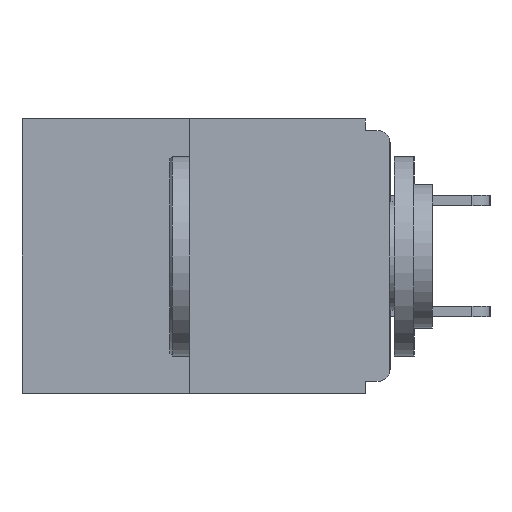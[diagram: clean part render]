
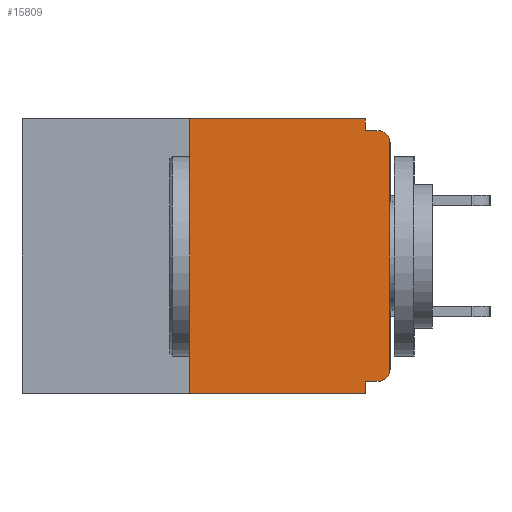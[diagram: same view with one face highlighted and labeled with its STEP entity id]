
A CAD part, left-side view. The second image highlights one B-rep face of the part: STEP entity #15809.
In plain terms, the highlighted planar face has unit normal (-1, 0, 0).
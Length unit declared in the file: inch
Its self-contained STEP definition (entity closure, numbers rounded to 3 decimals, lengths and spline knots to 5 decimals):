
#145 = VERTEX_POINT ( 'NONE', #18050 ) ;
#243 = VECTOR ( 'NONE', #1153, 39.37008 ) ;
#760 = CARTESIAN_POINT ( 'NONE',  ( 0., 0.015, -0.313 ) ) ;
#883 = AXIS2_PLACEMENT_3D ( 'NONE', #3754, #13693, #15143 ) ;
#996 = CARTESIAN_POINT ( 'NONE',  ( 0., 0.25, -0.343 ) ) ;
#1153 = DIRECTION ( 'NONE',  ( 0., -1., 0. ) ) ;
#1830 = AXIS2_PLACEMENT_3D ( 'NONE', #760, #5051, #13548 ) ;
#1889 = VECTOR ( 'NONE', #18510, 39.37008 ) ;
#1941 = CARTESIAN_POINT ( 'NONE',  ( 0., 0.46, 0. ) ) ;
#2300 = CARTESIAN_POINT ( 'NONE',  ( 0., 0., -0.328 ) ) ;
#2359 = EDGE_CURVE ( 'NONE', #15638, #13680, #3299, .T. ) ;
#2834 = CARTESIAN_POINT ( 'NONE',  ( 0., 0., 0. ) ) ;
#2894 = LINE ( 'NONE', #7055, #243 ) ;
#3003 = VERTEX_POINT ( 'NONE', #5854 ) ;
#3083 = CARTESIAN_POINT ( 'NONE',  ( 0., 0., -0.03 ) ) ;
#3299 = LINE ( 'NONE', #2300, #8972 ) ;
#3565 = EDGE_CURVE ( 'NONE', #4010, #8163, #9805, .T. ) ;
#3754 = CARTESIAN_POINT ( 'NONE',  ( 0., 0.015, -0.03 ) ) ;
#4010 = VERTEX_POINT ( 'NONE', #996 ) ;
#4571 = EDGE_CURVE ( 'NONE', #13680, #8163, #14696, .T. ) ;
#4770 = VERTEX_POINT ( 'NONE', #6457 ) ;
#4928 = DIRECTION ( 'NONE',  ( 0., 0., 1. ) ) ;
#5038 = ORIENTED_EDGE ( 'NONE', *, *, #4571, .F. ) ;
#5051 = DIRECTION ( 'NONE',  ( -1., 0., 0. ) ) ;
#5304 = LINE ( 'NONE', #11461, #16091 ) ;
#5854 = CARTESIAN_POINT ( 'NONE',  ( 0., 0.25, 0. ) ) ;
#6201 = FACE_OUTER_BOUND ( 'NONE', #9965, .T. ) ;
#6348 = CARTESIAN_POINT ( 'NONE',  ( 0., 0.031, -0.328 ) ) ;
#6443 = CIRCLE ( 'NONE', #883, 0.015 ) ;
#6457 = CARTESIAN_POINT ( 'NONE',  ( 0., 0.031, -0.015 ) ) ;
#6473 = ORIENTED_EDGE ( 'NONE', *, *, #14802, .T. ) ;
#6986 = ORIENTED_EDGE ( 'NONE', *, *, #7408, .F. ) ;
#7055 = CARTESIAN_POINT ( 'NONE',  ( 0., 0., -0.015 ) ) ;
#7408 = EDGE_CURVE ( 'NONE', #4010, #3003, #18420, .T. ) ;
#7419 = EDGE_CURVE ( 'NONE', #15638, #7931, #9023, .T. ) ;
#7622 = ORIENTED_EDGE ( 'NONE', *, *, #8423, .F. ) ;
#7807 = VECTOR ( 'NONE', #12452, 39.37008 ) ;
#7931 = VERTEX_POINT ( 'NONE', #12604 ) ;
#8163 = VERTEX_POINT ( 'NONE', #13456 ) ;
#8423 = EDGE_CURVE ( 'NONE', #4770, #145, #2894, .T. ) ;
#8503 = VERTEX_POINT ( 'NONE', #3083 ) ;
#8972 = VECTOR ( 'NONE', #16705, 39.37008 ) ;
#9023 = CIRCLE ( 'NONE', #1830, 0.015 ) ;
#9253 = DIRECTION ( 'NONE',  ( 0., 0., -1. ) ) ;
#9265 = ORIENTED_EDGE ( 'NONE', *, *, #10621, .F. ) ;
#9805 = LINE ( 'NONE', #14299, #16961 ) ;
#9965 = EDGE_LOOP ( 'NONE', ( #13039, #6986, #12338, #5038, #16274, #18297, #6473, #18188, #7622, #9265 ) ) ;
#10621 = EDGE_CURVE ( 'NONE', #16051, #4770, #5304, .T. ) ;
#10687 = CARTESIAN_POINT ( 'NONE',  ( 0., 0.25, 0. ) ) ;
#10936 = EDGE_CURVE ( 'NONE', #8503, #145, #6443, .T. ) ;
#11272 = AXIS2_PLACEMENT_3D ( 'NONE', #1941, #17867, #9253 ) ;
#11461 = CARTESIAN_POINT ( 'NONE',  ( 0., 0.031, 0. ) ) ;
#12081 = LINE ( 'NONE', #12509, #7807 ) ;
#12338 = ORIENTED_EDGE ( 'NONE', *, *, #3565, .T. ) ;
#12452 = DIRECTION ( 'NONE',  ( 0., -1., 0. ) ) ;
#12509 = CARTESIAN_POINT ( 'NONE',  ( 0., 0.46, 0. ) ) ;
#12538 = CARTESIAN_POINT ( 'NONE',  ( 0., 0.031, 0. ) ) ;
#12604 = CARTESIAN_POINT ( 'NONE',  ( 0., 0., -0.313 ) ) ;
#12689 = CARTESIAN_POINT ( 'NONE',  ( 0., 0.031, -0.343 ) ) ;
#12881 = DIRECTION ( 'NONE',  ( 0., 0., 1. ) ) ;
#13039 = ORIENTED_EDGE ( 'NONE', *, *, #14723, .F. ) ;
#13180 = LINE ( 'NONE', #2834, #14549 ) ;
#13456 = CARTESIAN_POINT ( 'NONE',  ( 0., 0.031, -0.343 ) ) ;
#13548 = DIRECTION ( 'NONE',  ( 0., 0., -1. ) ) ;
#13680 = VERTEX_POINT ( 'NONE', #6348 ) ;
#13693 = DIRECTION ( 'NONE',  ( -1., 0., 0. ) ) ;
#14240 = CARTESIAN_POINT ( 'NONE',  ( 0., 0.015, -0.328 ) ) ;
#14299 = CARTESIAN_POINT ( 'NONE',  ( 0., 0.46, -0.343 ) ) ;
#14526 = DIRECTION ( 'NONE',  ( 0., 0., -1. ) ) ;
#14549 = VECTOR ( 'NONE', #12881, 39.37008 ) ;
#14696 = LINE ( 'NONE', #12689, #1889 ) ;
#14723 = EDGE_CURVE ( 'NONE', #3003, #16051, #12081, .T. ) ;
#14802 = EDGE_CURVE ( 'NONE', #7931, #8503, #13180, .T. ) ;
#14878 = PLANE ( 'NONE',  #11272 ) ;
#15143 = DIRECTION ( 'NONE',  ( 0., 0., -1. ) ) ;
#15638 = VERTEX_POINT ( 'NONE', #14240 ) ;
#15687 = DIRECTION ( 'NONE',  ( 0., -1., 0. ) ) ;
#15809 = ADVANCED_FACE ( 'NONE', ( #6201 ), #14878, .F. ) ;
#16051 = VERTEX_POINT ( 'NONE', #12538 ) ;
#16091 = VECTOR ( 'NONE', #14526, 39.37008 ) ;
#16274 = ORIENTED_EDGE ( 'NONE', *, *, #2359, .F. ) ;
#16705 = DIRECTION ( 'NONE',  ( 0., 1., 0. ) ) ;
#16845 = VECTOR ( 'NONE', #4928, 39.37008 ) ;
#16961 = VECTOR ( 'NONE', #15687, 39.37008 ) ;
#17867 = DIRECTION ( 'NONE',  ( 1., 0., 0. ) ) ;
#18050 = CARTESIAN_POINT ( 'NONE',  ( 0., 0.015, -0.015 ) ) ;
#18188 = ORIENTED_EDGE ( 'NONE', *, *, #10936, .T. ) ;
#18297 = ORIENTED_EDGE ( 'NONE', *, *, #7419, .T. ) ;
#18420 = LINE ( 'NONE', #10687, #16845 ) ;
#18510 = DIRECTION ( 'NONE',  ( 0., 0., -1. ) ) ;
